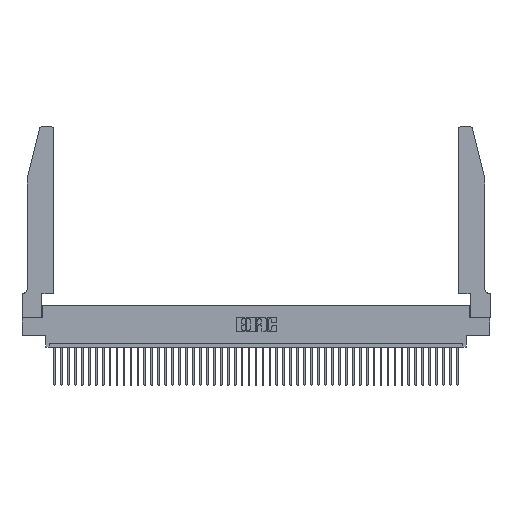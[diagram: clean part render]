
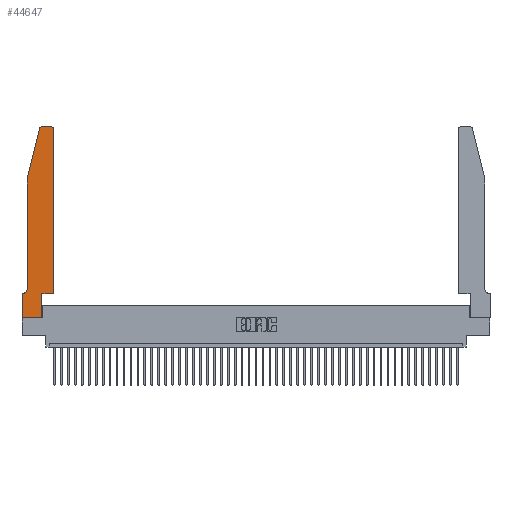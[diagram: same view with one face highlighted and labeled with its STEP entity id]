
A CAD part, top view. The second image highlights one B-rep face of the part: STEP entity #44647.
In plain terms, the highlighted planar face has unit normal (0, 0, 1).
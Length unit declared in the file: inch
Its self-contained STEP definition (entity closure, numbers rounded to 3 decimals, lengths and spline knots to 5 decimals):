
#590 = CARTESIAN_POINT ( 'NONE',  ( 0.0055, 0.35, 0.37 ) ) ;
#869 = VECTOR ( 'NONE', #8803, 39.37008 ) ;
#968 = VERTEX_POINT ( 'NONE', #5821 ) ;
#1142 = LINE ( 'NONE', #41687, #17654 ) ;
#1422 = EDGE_CURVE ( 'NONE', #10468, #40179, #34758, .T. ) ;
#1605 = VERTEX_POINT ( 'NONE', #46891 ) ;
#1834 = DIRECTION ( 'NONE',  ( 0., 0., 1. ) ) ;
#2937 = AXIS2_PLACEMENT_3D ( 'NONE', #14940, #40235, #18570 ) ;
#3525 = ORIENTED_EDGE ( 'NONE', *, *, #28606, .T. ) ;
#4855 = DIRECTION ( 'NONE',  ( 1., 0., 0. ) ) ;
#5015 = LINE ( 'NONE', #24684, #43028 ) ;
#5228 = DIRECTION ( 'NONE',  ( 0., 0., 1. ) ) ;
#5821 = CARTESIAN_POINT ( 'NONE',  ( 0.284, 2.75, 0.37 ) ) ;
#6517 = CARTESIAN_POINT ( 'NONE',  ( 0.4205, 2.75, 0.37 ) ) ;
#6622 = CARTESIAN_POINT ( 'NONE',  ( 0.25487, 2.72718, 0.37 ) ) ;
#6876 = CARTESIAN_POINT ( 'NONE',  ( 0., 0., 0.37 ) ) ;
#7683 = CIRCLE ( 'NONE', #18407, 0.07 ) ;
#8353 = CIRCLE ( 'NONE', #44607, 0.03 ) ;
#8803 = DIRECTION ( 'NONE',  ( 0., -1., 0. ) ) ;
#8875 = EDGE_CURVE ( 'NONE', #33007, #10468, #38037, .T. ) ;
#8979 = CARTESIAN_POINT ( 'NONE',  ( 0.4505, 2.72, 0.37 ) ) ;
#9609 = CARTESIAN_POINT ( 'NONE',  ( 0.0755, 2., 0.37 ) ) ;
#9833 = VECTOR ( 'NONE', #25185, 39.37008 ) ;
#9967 = VERTEX_POINT ( 'NONE', #27096 ) ;
#10468 = VERTEX_POINT ( 'NONE', #13255 ) ;
#10925 = EDGE_CURVE ( 'NONE', #1605, #33007, #5015, .T. ) ;
#11277 = CARTESIAN_POINT ( 'NONE',  ( 0.4505, 0.35, 0.37 ) ) ;
#11739 = CARTESIAN_POINT ( 'NONE',  ( 0.2865, 0.35, 0.37 ) ) ;
#11989 = CARTESIAN_POINT ( 'NONE',  ( 0.4505, 0.35, 0.37 ) ) ;
#12741 = DIRECTION ( 'NONE',  ( -1., 0., 0. ) ) ;
#12953 = ORIENTED_EDGE ( 'NONE', *, *, #40527, .T. ) ;
#13055 = CARTESIAN_POINT ( 'NONE',  ( 0.0755, 0.35, 0.37 ) ) ;
#13255 = CARTESIAN_POINT ( 'NONE',  ( 0.2865, 0., 0.37 ) ) ;
#14162 = VERTEX_POINT ( 'NONE', #8979 ) ;
#14696 = LINE ( 'NONE', #13055, #20892 ) ;
#14703 = ORIENTED_EDGE ( 'NONE', *, *, #43640, .T. ) ;
#14937 = VECTOR ( 'NONE', #41977, 39.37008 ) ;
#14940 = CARTESIAN_POINT ( 'NONE',  ( 0., 0.35, 0.37 ) ) ;
#16496 = VECTOR ( 'NONE', #4855, 39.37008 ) ;
#17639 = LINE ( 'NONE', #11989, #16496 ) ;
#17654 = VECTOR ( 'NONE', #28677, 39.37008 ) ;
#18223 = ORIENTED_EDGE ( 'NONE', *, *, #8875, .T. ) ;
#18407 = AXIS2_PLACEMENT_3D ( 'NONE', #41717, #34246, #12741 ) ;
#18426 = EDGE_CURVE ( 'NONE', #968, #28254, #8353, .T. ) ;
#18462 = LINE ( 'NONE', #9609, #41672 ) ;
#18570 = DIRECTION ( 'NONE',  ( 1., 0., 0. ) ) ;
#19438 = EDGE_CURVE ( 'NONE', #14162, #21422, #39958, .T. ) ;
#19560 = ORIENTED_EDGE ( 'NONE', *, *, #1422, .T. ) ;
#20892 = VECTOR ( 'NONE', #42322, 39.37008 ) ;
#21422 = VERTEX_POINT ( 'NONE', #6517 ) ;
#21593 = EDGE_CURVE ( 'NONE', #40179, #42872, #17639, .T. ) ;
#22020 = VERTEX_POINT ( 'NONE', #35430 ) ;
#24684 = CARTESIAN_POINT ( 'NONE',  ( 0., 0., 0.37 ) ) ;
#25070 = EDGE_CURVE ( 'NONE', #9967, #28823, #7683, .T. ) ;
#25177 = LINE ( 'NONE', #46882, #9833 ) ;
#25185 = DIRECTION ( 'NONE',  ( -1., 0., 0. ) ) ;
#26601 = DIRECTION ( 'NONE',  ( 1., 0., 0. ) ) ;
#27096 = CARTESIAN_POINT ( 'NONE',  ( 0.0755, 0.42, 0.37 ) ) ;
#27231 = CARTESIAN_POINT ( 'NONE',  ( 0.4205, 2.72, 0.37 ) ) ;
#27821 = VECTOR ( 'NONE', #28039, 39.37008 ) ;
#28039 = DIRECTION ( 'NONE',  ( 1., 0., 0. ) ) ;
#28175 = LINE ( 'NONE', #38265, #869 ) ;
#28194 = CARTESIAN_POINT ( 'NONE',  ( 0., 0., 0.37 ) ) ;
#28254 = VERTEX_POINT ( 'NONE', #6622 ) ;
#28606 = EDGE_CURVE ( 'NONE', #28254, #22020, #18462, .T. ) ;
#28677 = DIRECTION ( 'NONE',  ( 0., 1., 0. ) ) ;
#28681 = ORIENTED_EDGE ( 'NONE', *, *, #29233, .T. ) ;
#28823 = VERTEX_POINT ( 'NONE', #590 ) ;
#29233 = EDGE_CURVE ( 'NONE', #21422, #968, #25177, .T. ) ;
#31337 = DIRECTION ( 'NONE',  ( 0., -1., 0. ) ) ;
#31726 = EDGE_LOOP ( 'NONE', ( #28681, #40485, #3525, #14703, #40690, #39142, #38251, #18223, #19560, #43952, #12953, #32971 ) ) ;
#32194 = EDGE_CURVE ( 'NONE', #28823, #1605, #14696, .T. ) ;
#32808 = AXIS2_PLACEMENT_3D ( 'NONE', #27231, #1834, #43089 ) ;
#32971 = ORIENTED_EDGE ( 'NONE', *, *, #19438, .T. ) ;
#33007 = VERTEX_POINT ( 'NONE', #6876 ) ;
#34246 = DIRECTION ( 'NONE',  ( 0., 0., -1. ) ) ;
#34758 = LINE ( 'NONE', #45294, #14937 ) ;
#34944 = DIRECTION ( 'NONE',  ( -0.239, -0.971, 0. ) ) ;
#35430 = CARTESIAN_POINT ( 'NONE',  ( 0.0755, 2., 0.37 ) ) ;
#38037 = LINE ( 'NONE', #28194, #27821 ) ;
#38251 = ORIENTED_EDGE ( 'NONE', *, *, #10925, .T. ) ;
#38265 = CARTESIAN_POINT ( 'NONE',  ( 0.0755, 2., 0.37 ) ) ;
#39142 = ORIENTED_EDGE ( 'NONE', *, *, #32194, .T. ) ;
#39356 = FACE_OUTER_BOUND ( 'NONE', #31726, .T. ) ;
#39958 = CIRCLE ( 'NONE', #32808, 0.03 ) ;
#40179 = VERTEX_POINT ( 'NONE', #11739 ) ;
#40235 = DIRECTION ( 'NONE',  ( 0., 0., 1. ) ) ;
#40485 = ORIENTED_EDGE ( 'NONE', *, *, #18426, .T. ) ;
#40527 = EDGE_CURVE ( 'NONE', #42872, #14162, #1142, .T. ) ;
#40554 = PLANE ( 'NONE',  #2937 ) ;
#40690 = ORIENTED_EDGE ( 'NONE', *, *, #25070, .T. ) ;
#41672 = VECTOR ( 'NONE', #34944, 39.37008 ) ;
#41687 = CARTESIAN_POINT ( 'NONE',  ( 0.4505, 0.35, 0.37 ) ) ;
#41717 = CARTESIAN_POINT ( 'NONE',  ( 0.0055, 0.42, 0.37 ) ) ;
#41977 = DIRECTION ( 'NONE',  ( 0., 1., 0. ) ) ;
#42322 = DIRECTION ( 'NONE',  ( -1., 0., 0. ) ) ;
#42872 = VERTEX_POINT ( 'NONE', #11277 ) ;
#43028 = VECTOR ( 'NONE', #31337, 39.37008 ) ;
#43089 = DIRECTION ( 'NONE',  ( 1., 0., 0. ) ) ;
#43640 = EDGE_CURVE ( 'NONE', #22020, #9967, #28175, .T. ) ;
#43952 = ORIENTED_EDGE ( 'NONE', *, *, #21593, .T. ) ;
#44607 = AXIS2_PLACEMENT_3D ( 'NONE', #44971, #5228, #26601 ) ;
#44647 = ADVANCED_FACE ( 'NONE', ( #39356 ), #40554, .T. ) ;
#44971 = CARTESIAN_POINT ( 'NONE',  ( 0.284, 2.72, 0.37 ) ) ;
#45294 = CARTESIAN_POINT ( 'NONE',  ( 0.2865, 0.35, 0.37 ) ) ;
#46882 = CARTESIAN_POINT ( 'NONE',  ( 0.2605, 2.75, 0.37 ) ) ;
#46891 = CARTESIAN_POINT ( 'NONE',  ( 0., 0.35, 0.37 ) ) ;
